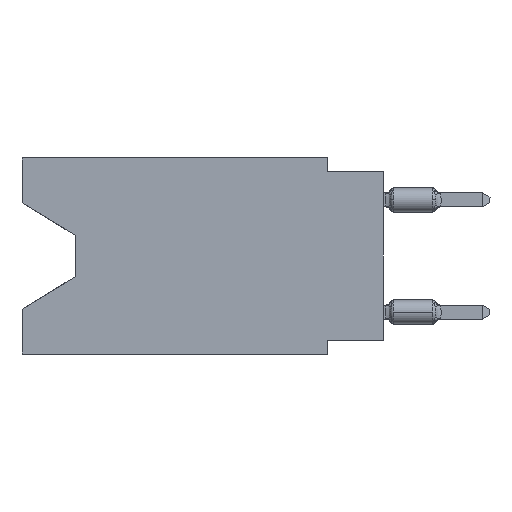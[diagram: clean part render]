
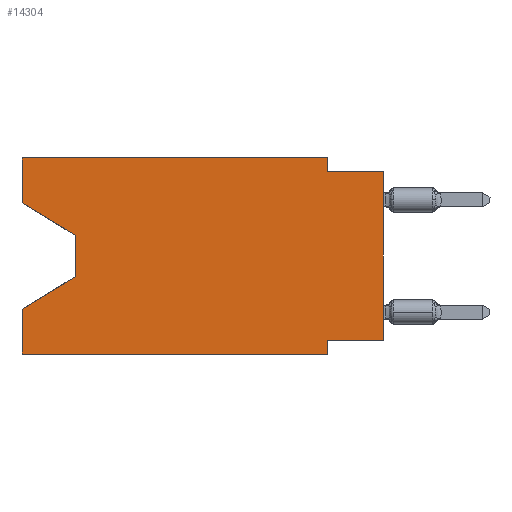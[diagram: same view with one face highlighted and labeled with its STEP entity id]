
A CAD part, left-side view. The second image highlights one B-rep face of the part: STEP entity #14304.
In plain terms, the highlighted planar face has unit normal (-1, 0, 0).
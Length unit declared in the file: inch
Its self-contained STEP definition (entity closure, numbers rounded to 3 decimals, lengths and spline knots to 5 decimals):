
#50 = DIRECTION ( 'NONE',  ( 0., 0., -1. ) ) ;
#98 = ORIENTED_EDGE ( 'NONE', *, *, #18060, .T. ) ;
#774 = EDGE_CURVE ( 'NONE', #9232, #5927, #12972, .T. ) ;
#783 = CARTESIAN_POINT ( 'NONE',  ( 0., 0.55, -0.212 ) ) ;
#784 = DIRECTION ( 'NONE',  ( 0., -1., 0. ) ) ;
#866 = EDGE_LOOP ( 'NONE', ( #98, #9211, #5832, #10652, #16088, #12325, #6273, #12029, #1248, #17914, #14129, #12684 ) ) ;
#886 = CARTESIAN_POINT ( 'NONE',  ( 0., 0., -0.025 ) ) ;
#1067 = VERTEX_POINT ( 'NONE', #13216 ) ;
#1144 = EDGE_CURVE ( 'NONE', #16660, #7685, #18757, .T. ) ;
#1164 = EDGE_CURVE ( 'NONE', #5733, #9232, #3928, .T. ) ;
#1248 = ORIENTED_EDGE ( 'NONE', *, *, #774, .F. ) ;
#1605 = EDGE_CURVE ( 'NONE', #18792, #16807, #15939, .T. ) ;
#2884 = LINE ( 'NONE', #17943, #13159 ) ;
#3306 = CARTESIAN_POINT ( 'NONE',  ( 0., 0.645, 0. ) ) ;
#3395 = CARTESIAN_POINT ( 'NONE',  ( 0., 0.645, 0. ) ) ;
#3522 = VERTEX_POINT ( 'NONE', #8681 ) ;
#3928 = LINE ( 'NONE', #5243, #20005 ) ;
#3933 = VERTEX_POINT ( 'NONE', #7697 ) ;
#5032 = VECTOR ( 'NONE', #9766, 39.37008 ) ;
#5243 = CARTESIAN_POINT ( 'NONE',  ( 0., 0.1, 0. ) ) ;
#5311 = CARTESIAN_POINT ( 'NONE',  ( 0., 0.1, 0. ) ) ;
#5453 = CARTESIAN_POINT ( 'NONE',  ( 0., 0.645, 0. ) ) ;
#5465 = EDGE_CURVE ( 'NONE', #7685, #16807, #15259, .T. ) ;
#5733 = VERTEX_POINT ( 'NONE', #5311 ) ;
#5771 = VECTOR ( 'NONE', #15174, 39.37008 ) ;
#5832 = ORIENTED_EDGE ( 'NONE', *, *, #9122, .T. ) ;
#5927 = VERTEX_POINT ( 'NONE', #886 ) ;
#6273 = ORIENTED_EDGE ( 'NONE', *, *, #1144, .F. ) ;
#6577 = LINE ( 'NONE', #3395, #15622 ) ;
#7526 = DIRECTION ( 'NONE',  ( 0., -1., 0. ) ) ;
#7685 = VERTEX_POINT ( 'NONE', #18227 ) ;
#7697 = CARTESIAN_POINT ( 'NONE',  ( 0., 0.55, -0.138 ) ) ;
#7872 = CARTESIAN_POINT ( 'NONE',  ( 0., 0.1, -0.35 ) ) ;
#8197 = CARTESIAN_POINT ( 'NONE',  ( 0., 0.645, -0.08025 ) ) ;
#8429 = CARTESIAN_POINT ( 'NONE',  ( 0., 0.645, 0. ) ) ;
#8453 = VECTOR ( 'NONE', #18715, 39.37008 ) ;
#8625 = EDGE_CURVE ( 'NONE', #16660, #5927, #10479, .T. ) ;
#8681 = CARTESIAN_POINT ( 'NONE',  ( 0., 0.55, -0.212 ) ) ;
#9122 = EDGE_CURVE ( 'NONE', #3522, #18544, #10846, .T. ) ;
#9211 = ORIENTED_EDGE ( 'NONE', *, *, #14363, .T. ) ;
#9232 = VERTEX_POINT ( 'NONE', #19383 ) ;
#9766 = DIRECTION ( 'NONE',  ( 0., -1., 0. ) ) ;
#9972 = VECTOR ( 'NONE', #11982, 39.37008 ) ;
#10375 = EDGE_CURVE ( 'NONE', #19469, #5733, #2884, .T. ) ;
#10388 = VECTOR ( 'NONE', #19739, 39.37008 ) ;
#10419 = PLANE ( 'NONE',  #15967 ) ;
#10479 = LINE ( 'NONE', #17256, #15179 ) ;
#10524 = FACE_OUTER_BOUND ( 'NONE', #866, .T. ) ;
#10633 = LINE ( 'NONE', #15285, #11001 ) ;
#10652 = ORIENTED_EDGE ( 'NONE', *, *, #13731, .F. ) ;
#10846 = LINE ( 'NONE', #783, #15906 ) ;
#11001 = VECTOR ( 'NONE', #17412, 39.37008 ) ;
#11982 = DIRECTION ( 'NONE',  ( 0., 1., 0. ) ) ;
#12029 = ORIENTED_EDGE ( 'NONE', *, *, #8625, .T. ) ;
#12070 = DIRECTION ( 'NONE',  ( 1., 0., 0. ) ) ;
#12325 = ORIENTED_EDGE ( 'NONE', *, *, #5465, .F. ) ;
#12684 = ORIENTED_EDGE ( 'NONE', *, *, #12733, .F. ) ;
#12733 = EDGE_CURVE ( 'NONE', #1067, #19469, #18529, .T. ) ;
#12972 = LINE ( 'NONE', #14639, #5032 ) ;
#13159 = VECTOR ( 'NONE', #7526, 39.37008 ) ;
#13216 = CARTESIAN_POINT ( 'NONE',  ( 0., 0.645, -0.08025 ) ) ;
#13606 = CARTESIAN_POINT ( 'NONE',  ( 0., 0.1, -0.35 ) ) ;
#13630 = DIRECTION ( 'NONE',  ( 0., 0., -1. ) ) ;
#13731 = EDGE_CURVE ( 'NONE', #18792, #18544, #6577, .T. ) ;
#14129 = ORIENTED_EDGE ( 'NONE', *, *, #10375, .F. ) ;
#14304 = ADVANCED_FACE ( 'NONE', ( #10524 ), #10419, .F. ) ;
#14363 = EDGE_CURVE ( 'NONE', #3933, #3522, #10633, .T. ) ;
#14639 = CARTESIAN_POINT ( 'NONE',  ( 0., 0., -0.025 ) ) ;
#14846 = LINE ( 'NONE', #8197, #10388 ) ;
#15174 = DIRECTION ( 'NONE',  ( 0., 0., 1. ) ) ;
#15177 = CARTESIAN_POINT ( 'NONE',  ( 0., 0., -0.325 ) ) ;
#15179 = VECTOR ( 'NONE', #21012, 39.37008 ) ;
#15259 = LINE ( 'NONE', #13606, #8453 ) ;
#15285 = CARTESIAN_POINT ( 'NONE',  ( 0., 0.55, -0.138 ) ) ;
#15622 = VECTOR ( 'NONE', #20000, 39.37008 ) ;
#15906 = VECTOR ( 'NONE', #19492, 39.37008 ) ;
#15939 = LINE ( 'NONE', #19385, #16422 ) ;
#15967 = AXIS2_PLACEMENT_3D ( 'NONE', #5453, #12070, #13630 ) ;
#16088 = ORIENTED_EDGE ( 'NONE', *, *, #1605, .T. ) ;
#16422 = VECTOR ( 'NONE', #784, 39.37008 ) ;
#16660 = VERTEX_POINT ( 'NONE', #15177 ) ;
#16807 = VERTEX_POINT ( 'NONE', #7872 ) ;
#17256 = CARTESIAN_POINT ( 'NONE',  ( 0., 0., 0. ) ) ;
#17317 = CARTESIAN_POINT ( 'NONE',  ( 0., 0., -0.325 ) ) ;
#17412 = DIRECTION ( 'NONE',  ( 0., 0., -1. ) ) ;
#17628 = CARTESIAN_POINT ( 'NONE',  ( 0., 0.645, -0.35 ) ) ;
#17914 = ORIENTED_EDGE ( 'NONE', *, *, #1164, .F. ) ;
#17943 = CARTESIAN_POINT ( 'NONE',  ( 0., 0.645, 0. ) ) ;
#18060 = EDGE_CURVE ( 'NONE', #1067, #3933, #14846, .T. ) ;
#18227 = CARTESIAN_POINT ( 'NONE',  ( 0., 0.1, -0.325 ) ) ;
#18529 = LINE ( 'NONE', #8429, #5771 ) ;
#18544 = VERTEX_POINT ( 'NONE', #19605 ) ;
#18715 = DIRECTION ( 'NONE',  ( 0., 0., -1. ) ) ;
#18757 = LINE ( 'NONE', #17317, #9972 ) ;
#18792 = VERTEX_POINT ( 'NONE', #17628 ) ;
#19383 = CARTESIAN_POINT ( 'NONE',  ( 0., 0.1, -0.025 ) ) ;
#19385 = CARTESIAN_POINT ( 'NONE',  ( 0., 0.645, -0.35 ) ) ;
#19469 = VERTEX_POINT ( 'NONE', #3306 ) ;
#19492 = DIRECTION ( 'NONE',  ( 0., 0.855, -0.519 ) ) ;
#19605 = CARTESIAN_POINT ( 'NONE',  ( 0., 0.645, -0.26975 ) ) ;
#19739 = DIRECTION ( 'NONE',  ( 0., -0.855, -0.519 ) ) ;
#20000 = DIRECTION ( 'NONE',  ( 0., 0., 1. ) ) ;
#20005 = VECTOR ( 'NONE', #50, 39.37008 ) ;
#21012 = DIRECTION ( 'NONE',  ( 0., 0., 1. ) ) ;
